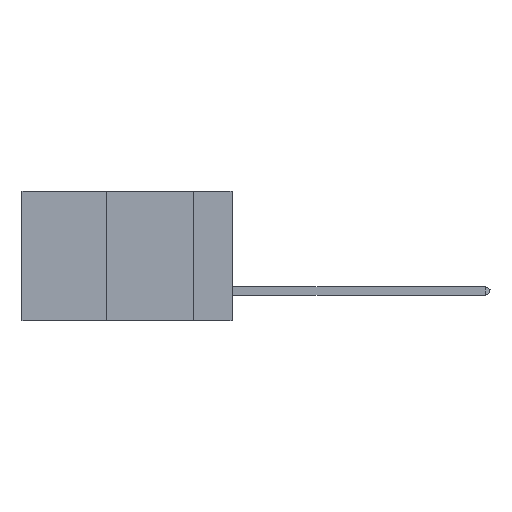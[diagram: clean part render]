
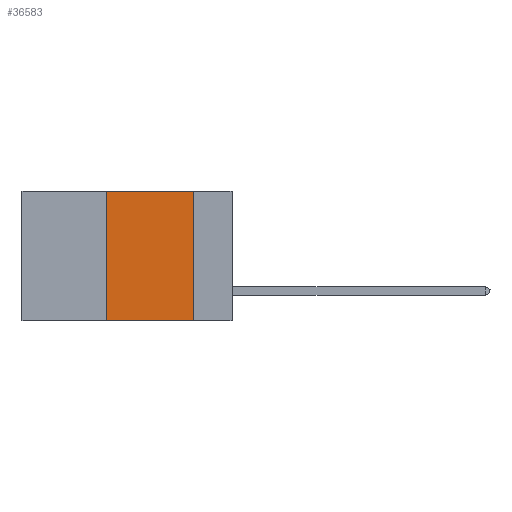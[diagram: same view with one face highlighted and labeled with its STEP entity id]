
A CAD part, left-side view. The second image highlights one B-rep face of the part: STEP entity #36583.
In plain terms, the highlighted planar face has unit normal (-1, 0, 0).
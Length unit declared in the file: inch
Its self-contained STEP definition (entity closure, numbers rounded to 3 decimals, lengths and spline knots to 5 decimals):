
#586 = DIRECTION ( 'NONE',  ( 1., 0., 0. ) ) ;
#749 = PLANE ( 'NONE',  #33517 ) ;
#1067 = DIRECTION ( 'NONE',  ( 0., 0., -1. ) ) ;
#1320 = FACE_OUTER_BOUND ( 'NONE', #36223, .T. ) ;
#2469 = VECTOR ( 'NONE', #46563, 39.37008 ) ;
#6486 = VERTEX_POINT ( 'NONE', #23910 ) ;
#7433 = ORIENTED_EDGE ( 'NONE', *, *, #28188, .F. ) ;
#7655 = CARTESIAN_POINT ( 'NONE',  ( 0., 0.36, 0. ) ) ;
#10037 = ORIENTED_EDGE ( 'NONE', *, *, #46645, .F. ) ;
#10166 = VERTEX_POINT ( 'NONE', #7655 ) ;
#11023 = CARTESIAN_POINT ( 'NONE',  ( 0., 0.36, 0. ) ) ;
#12927 = VECTOR ( 'NONE', #37964, 39.37008 ) ;
#15323 = LINE ( 'NONE', #11023, #29787 ) ;
#18244 = CARTESIAN_POINT ( 'NONE',  ( 0., 0.11, 0. ) ) ;
#18971 = VERTEX_POINT ( 'NONE', #36985 ) ;
#20393 = ORIENTED_EDGE ( 'NONE', *, *, #34175, .F. ) ;
#23333 = EDGE_CURVE ( 'NONE', #44409, #6486, #39729, .T. ) ;
#23910 = CARTESIAN_POINT ( 'NONE',  ( 0., 0.11, -0.37 ) ) ;
#23932 = ORIENTED_EDGE ( 'NONE', *, *, #23333, .T. ) ;
#28188 = EDGE_CURVE ( 'NONE', #18971, #6486, #33025, .T. ) ;
#28486 = CARTESIAN_POINT ( 'NONE',  ( 0., 0.6, -0.37 ) ) ;
#29125 = LINE ( 'NONE', #34233, #12927 ) ;
#29787 = VECTOR ( 'NONE', #40407, 39.37008 ) ;
#29926 = CARTESIAN_POINT ( 'NONE',  ( 0., 0.36, -0.37 ) ) ;
#30029 = CARTESIAN_POINT ( 'NONE',  ( 0., 0.6, 0. ) ) ;
#32819 = DIRECTION ( 'NONE',  ( 0., -1., 0. ) ) ;
#33025 = LINE ( 'NONE', #18244, #2469 ) ;
#33517 = AXIS2_PLACEMENT_3D ( 'NONE', #30029, #586, #1067 ) ;
#34175 = EDGE_CURVE ( 'NONE', #44409, #10166, #15323, .T. ) ;
#34233 = CARTESIAN_POINT ( 'NONE',  ( 0., 0.6, 0. ) ) ;
#36223 = EDGE_LOOP ( 'NONE', ( #7433, #10037, #20393, #23932 ) ) ;
#36583 = ADVANCED_FACE ( 'NONE', ( #1320 ), #749, .F. ) ;
#36985 = CARTESIAN_POINT ( 'NONE',  ( 0., 0.11, 0. ) ) ;
#37964 = DIRECTION ( 'NONE',  ( 0., -1., 0. ) ) ;
#39729 = LINE ( 'NONE', #28486, #46026 ) ;
#40407 = DIRECTION ( 'NONE',  ( 0., 0., 1. ) ) ;
#44409 = VERTEX_POINT ( 'NONE', #29926 ) ;
#46026 = VECTOR ( 'NONE', #32819, 39.37008 ) ;
#46563 = DIRECTION ( 'NONE',  ( 0., 0., -1. ) ) ;
#46645 = EDGE_CURVE ( 'NONE', #10166, #18971, #29125, .T. ) ;
